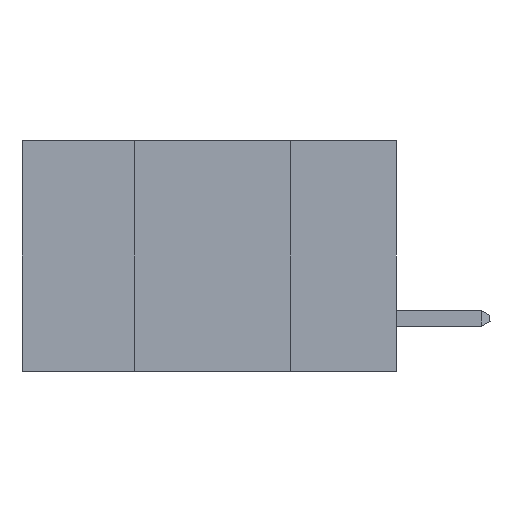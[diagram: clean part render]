
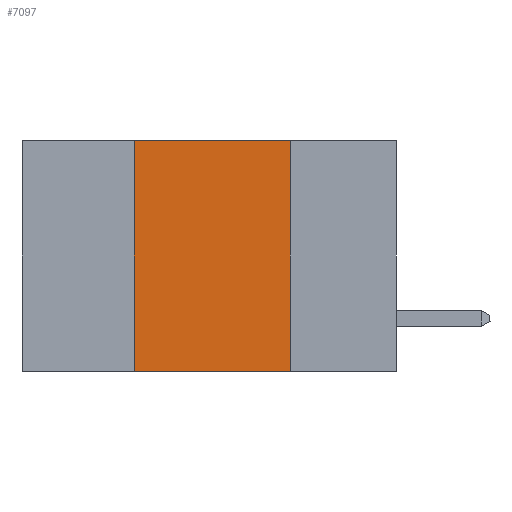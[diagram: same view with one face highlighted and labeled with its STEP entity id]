
A CAD part, left-side view. The second image highlights one B-rep face of the part: STEP entity #7097.
In plain terms, the highlighted planar face has unit normal (-1, 0, 0).
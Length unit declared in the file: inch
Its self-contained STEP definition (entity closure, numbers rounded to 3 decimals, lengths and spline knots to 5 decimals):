
#1026 = PLANE ( 'NONE',  #12958 ) ;
#1061 = CARTESIAN_POINT ( 'NONE',  ( 0., 0.42, 0. ) ) ;
#1176 = EDGE_CURVE ( 'NONE', #2082, #8935, #21193, .T. ) ;
#1995 = DIRECTION ( 'NONE',  ( 1., 0., 0. ) ) ;
#2082 = VERTEX_POINT ( 'NONE', #16760 ) ;
#2230 = ORIENTED_EDGE ( 'NONE', *, *, #7053, .F. ) ;
#2523 = ORIENTED_EDGE ( 'NONE', *, *, #1176, .F. ) ;
#2895 = CARTESIAN_POINT ( 'NONE',  ( 0., 0.17, -0.37 ) ) ;
#3444 = CARTESIAN_POINT ( 'NONE',  ( 0., 0.17, 0. ) ) ;
#3836 = EDGE_LOOP ( 'NONE', ( #2523, #17595, #2230, #12507 ) ) ;
#5670 = CARTESIAN_POINT ( 'NONE',  ( 0., 0.6, 0. ) ) ;
#6187 = CARTESIAN_POINT ( 'NONE',  ( 0., 0.42, -0.37 ) ) ;
#7053 = EDGE_CURVE ( 'NONE', #10631, #13622, #20300, .T. ) ;
#7097 = ADVANCED_FACE ( 'NONE', ( #13823 ), #1026, .F. ) ;
#7424 = DIRECTION ( 'NONE',  ( 0., 0., -1. ) ) ;
#7671 = DIRECTION ( 'NONE',  ( 0., -1., 0. ) ) ;
#8935 = VERTEX_POINT ( 'NONE', #2895 ) ;
#9323 = DIRECTION ( 'NONE',  ( 0., 0., 1. ) ) ;
#10142 = LINE ( 'NONE', #13506, #14600 ) ;
#10631 = VERTEX_POINT ( 'NONE', #6187 ) ;
#12100 = LINE ( 'NONE', #22440, #22775 ) ;
#12507 = ORIENTED_EDGE ( 'NONE', *, *, #16756, .T. ) ;
#12651 = EDGE_CURVE ( 'NONE', #13622, #2082, #12100, .T. ) ;
#12958 = AXIS2_PLACEMENT_3D ( 'NONE', #5670, #1995, #13323 ) ;
#13323 = DIRECTION ( 'NONE',  ( 0., 0., -1. ) ) ;
#13506 = CARTESIAN_POINT ( 'NONE',  ( 0., 0.6, -0.37 ) ) ;
#13622 = VERTEX_POINT ( 'NONE', #1061 ) ;
#13823 = FACE_OUTER_BOUND ( 'NONE', #3836, .T. ) ;
#14600 = VECTOR ( 'NONE', #7671, 39.37008 ) ;
#15284 = VECTOR ( 'NONE', #9323, 39.37008 ) ;
#15301 = CARTESIAN_POINT ( 'NONE',  ( 0., 0.42, 0. ) ) ;
#16756 = EDGE_CURVE ( 'NONE', #10631, #8935, #10142, .T. ) ;
#16760 = CARTESIAN_POINT ( 'NONE',  ( 0., 0.17, 0. ) ) ;
#17595 = ORIENTED_EDGE ( 'NONE', *, *, #12651, .F. ) ;
#18551 = DIRECTION ( 'NONE',  ( 0., -1., 0. ) ) ;
#20300 = LINE ( 'NONE', #15301, #15284 ) ;
#20601 = VECTOR ( 'NONE', #7424, 39.37008 ) ;
#21193 = LINE ( 'NONE', #3444, #20601 ) ;
#22440 = CARTESIAN_POINT ( 'NONE',  ( 0., 0.6, 0. ) ) ;
#22775 = VECTOR ( 'NONE', #18551, 39.37008 ) ;
